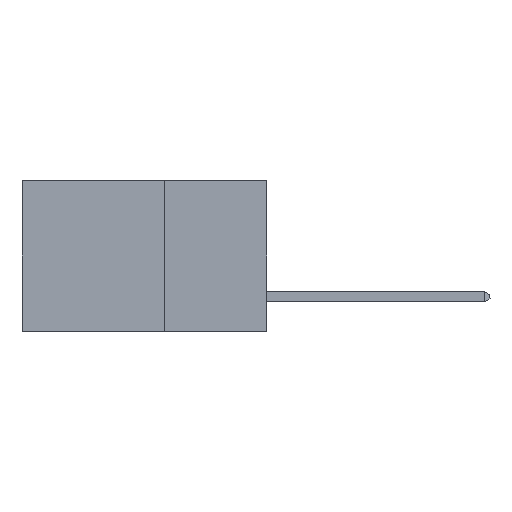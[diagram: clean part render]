
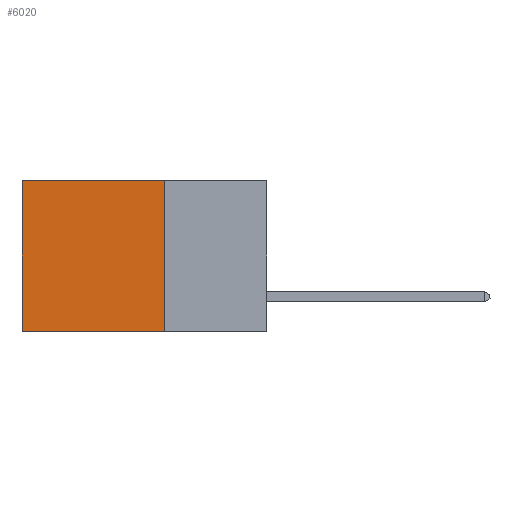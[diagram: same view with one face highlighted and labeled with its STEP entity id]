
A CAD part, left-side view. The second image highlights one B-rep face of the part: STEP entity #6020.
In plain terms, the highlighted planar face has unit normal (-1, 0, 0).
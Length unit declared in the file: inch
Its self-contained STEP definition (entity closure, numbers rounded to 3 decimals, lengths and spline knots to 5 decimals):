
#327 = ORIENTED_EDGE ( 'NONE', *, *, #8087, .F. ) ;
#447 = ORIENTED_EDGE ( 'NONE', *, *, #3114, .T. ) ;
#1374 = VECTOR ( 'NONE', #5598, 39.37008 ) ;
#2181 = FACE_OUTER_BOUND ( 'NONE', #15154, .T. ) ;
#2440 = VERTEX_POINT ( 'NONE', #7690 ) ;
#3114 = EDGE_CURVE ( 'NONE', #2440, #20950, #9588, .T. ) ;
#3699 = DIRECTION ( 'NONE',  ( 1., 0., 0. ) ) ;
#3701 = CARTESIAN_POINT ( 'NONE',  ( 0.2875, 0.25, 0. ) ) ;
#4937 = VECTOR ( 'NONE', #20944, 39.37008 ) ;
#5598 = DIRECTION ( 'NONE',  ( 0., 0., -1. ) ) ;
#5928 = AXIS2_PLACEMENT_3D ( 'NONE', #12981, #3699, #16543 ) ;
#6020 = ADVANCED_FACE ( 'NONE', ( #2181 ), #23613, .F. ) ;
#6403 = CARTESIAN_POINT ( 'NONE',  ( 0.2875, 0.25, 0. ) ) ;
#7690 = CARTESIAN_POINT ( 'NONE',  ( 0.2875, 0.6, 0. ) ) ;
#8057 = CARTESIAN_POINT ( 'NONE',  ( 0.2875, 0.6, 0. ) ) ;
#8087 = EDGE_CURVE ( 'NONE', #11838, #20950, #18212, .T. ) ;
#9418 = DIRECTION ( 'NONE',  ( 0., 1., 0. ) ) ;
#9588 = LINE ( 'NONE', #8057, #19164 ) ;
#11260 = CARTESIAN_POINT ( 'NONE',  ( 0.2875, 0.25, -0.37 ) ) ;
#11826 = VERTEX_POINT ( 'NONE', #18961 ) ;
#11838 = VERTEX_POINT ( 'NONE', #19040 ) ;
#12284 = EDGE_CURVE ( 'NONE', #11826, #11838, #15502, .T. ) ;
#12981 = CARTESIAN_POINT ( 'NONE',  ( 0.2875, 0.25, 0. ) ) ;
#13587 = ORIENTED_EDGE ( 'NONE', *, *, #12284, .F. ) ;
#13817 = EDGE_CURVE ( 'NONE', #11826, #2440, #15318, .T. ) ;
#15154 = EDGE_LOOP ( 'NONE', ( #447, #327, #13587, #18379 ) ) ;
#15318 = LINE ( 'NONE', #6403, #4937 ) ;
#15502 = LINE ( 'NONE', #3701, #1374 ) ;
#16543 = DIRECTION ( 'NONE',  ( 0., 0., -1. ) ) ;
#16835 = CARTESIAN_POINT ( 'NONE',  ( 0.2875, 0.6, -0.37 ) ) ;
#18212 = LINE ( 'NONE', #11260, #22424 ) ;
#18379 = ORIENTED_EDGE ( 'NONE', *, *, #13817, .T. ) ;
#18961 = CARTESIAN_POINT ( 'NONE',  ( 0.2875, 0.25, 0. ) ) ;
#19040 = CARTESIAN_POINT ( 'NONE',  ( 0.2875, 0.25, -0.37 ) ) ;
#19164 = VECTOR ( 'NONE', #22514, 39.37008 ) ;
#20944 = DIRECTION ( 'NONE',  ( 0., 1., 0. ) ) ;
#20950 = VERTEX_POINT ( 'NONE', #16835 ) ;
#22424 = VECTOR ( 'NONE', #9418, 39.37008 ) ;
#22514 = DIRECTION ( 'NONE',  ( 0., 0., -1. ) ) ;
#23613 = PLANE ( 'NONE',  #5928 ) ;
